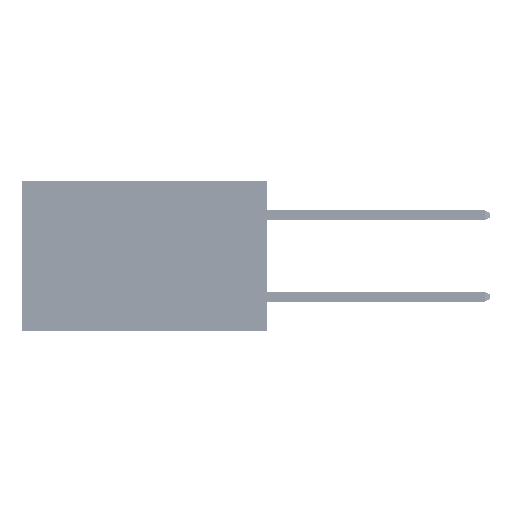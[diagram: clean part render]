
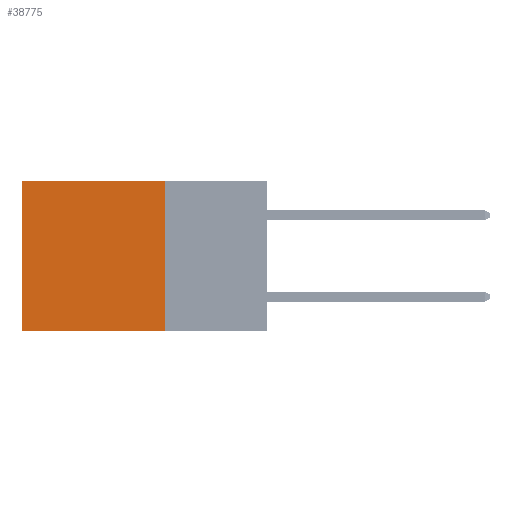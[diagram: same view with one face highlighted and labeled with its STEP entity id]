
A CAD part, left-side view. The second image highlights one B-rep face of the part: STEP entity #38775.
In plain terms, the highlighted planar face has unit normal (-1, 0, 0).
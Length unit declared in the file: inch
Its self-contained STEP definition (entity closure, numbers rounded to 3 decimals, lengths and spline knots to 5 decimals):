
#8 = EDGE_CURVE ( 'NONE', #10401, #7647, #3422, .T. ) ;
#865 = ORIENTED_EDGE ( 'NONE', *, *, #18846, .F. ) ;
#1710 = ORIENTED_EDGE ( 'NONE', *, *, #29666, .T. ) ;
#2060 = CARTESIAN_POINT ( 'NONE',  ( 0.2875, 0.25, 0. ) ) ;
#3191 = PLANE ( 'NONE',  #30597 ) ;
#3422 = LINE ( 'NONE', #29058, #48594 ) ;
#7621 = CARTESIAN_POINT ( 'NONE',  ( 0.2875, 0.6, -0.37 ) ) ;
#7647 = VERTEX_POINT ( 'NONE', #7621 ) ;
#8923 = VERTEX_POINT ( 'NONE', #20982 ) ;
#10401 = VERTEX_POINT ( 'NONE', #25858 ) ;
#10453 = EDGE_LOOP ( 'NONE', ( #30808, #865, #50979, #1710 ) ) ;
#11886 = LINE ( 'NONE', #29743, #42244 ) ;
#14946 = DIRECTION ( 'NONE',  ( 0., 0., -1. ) ) ;
#18846 = EDGE_CURVE ( 'NONE', #8923, #7647, #46385, .T. ) ;
#20982 = CARTESIAN_POINT ( 'NONE',  ( 0.2875, 0.25, -0.37 ) ) ;
#24082 = VECTOR ( 'NONE', #29669, 39.37008 ) ;
#25395 = EDGE_CURVE ( 'NONE', #26773, #8923, #39577, .T. ) ;
#25858 = CARTESIAN_POINT ( 'NONE',  ( 0.2875, 0.6, 0. ) ) ;
#26773 = VERTEX_POINT ( 'NONE', #38481 ) ;
#29058 = CARTESIAN_POINT ( 'NONE',  ( 0.2875, 0.6, 0. ) ) ;
#29396 = DIRECTION ( 'NONE',  ( 0., 1., 0. ) ) ;
#29590 = DIRECTION ( 'NONE',  ( 0., 0., -1. ) ) ;
#29666 = EDGE_CURVE ( 'NONE', #26773, #10401, #11886, .T. ) ;
#29669 = DIRECTION ( 'NONE',  ( 0., 0., -1. ) ) ;
#29743 = CARTESIAN_POINT ( 'NONE',  ( 0.2875, 0.25, 0. ) ) ;
#30597 = AXIS2_PLACEMENT_3D ( 'NONE', #43289, #35135, #14946 ) ;
#30808 = ORIENTED_EDGE ( 'NONE', *, *, #8, .T. ) ;
#32115 = VECTOR ( 'NONE', #46674, 39.37008 ) ;
#35135 = DIRECTION ( 'NONE',  ( 1., 0., 0. ) ) ;
#38481 = CARTESIAN_POINT ( 'NONE',  ( 0.2875, 0.25, 0. ) ) ;
#38775 = ADVANCED_FACE ( 'NONE', ( #49087 ), #3191, .F. ) ;
#39577 = LINE ( 'NONE', #2060, #24082 ) ;
#42244 = VECTOR ( 'NONE', #29396, 39.37008 ) ;
#43289 = CARTESIAN_POINT ( 'NONE',  ( 0.2875, 0.25, 0. ) ) ;
#46385 = LINE ( 'NONE', #50131, #32115 ) ;
#46674 = DIRECTION ( 'NONE',  ( 0., 1., 0. ) ) ;
#48594 = VECTOR ( 'NONE', #29590, 39.37008 ) ;
#49087 = FACE_OUTER_BOUND ( 'NONE', #10453, .T. ) ;
#50131 = CARTESIAN_POINT ( 'NONE',  ( 0.2875, 0.25, -0.37 ) ) ;
#50979 = ORIENTED_EDGE ( 'NONE', *, *, #25395, .F. ) ;
